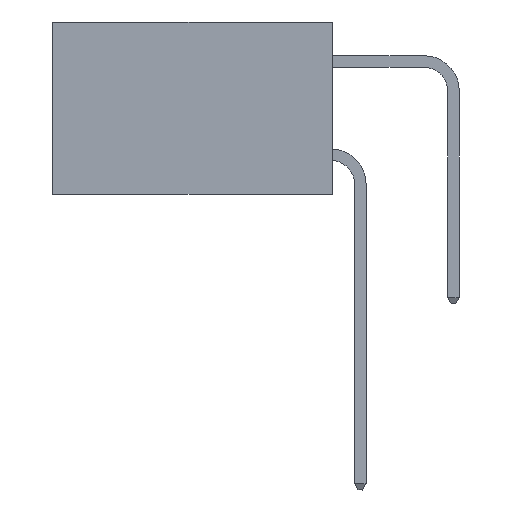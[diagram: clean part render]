
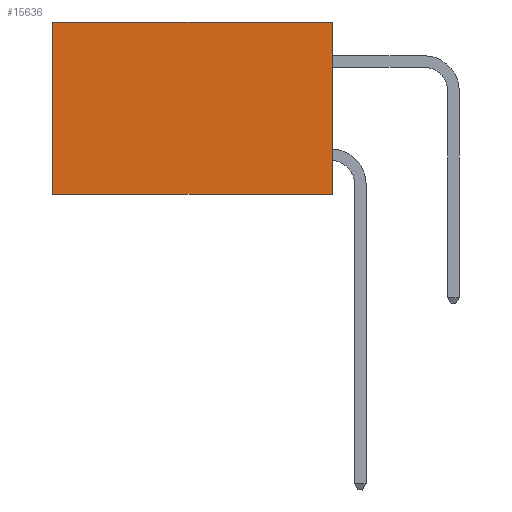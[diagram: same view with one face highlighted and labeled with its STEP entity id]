
A CAD part, left-side view. The second image highlights one B-rep face of the part: STEP entity #15636.
In plain terms, the highlighted planar face has unit normal (-1, 0, 0).
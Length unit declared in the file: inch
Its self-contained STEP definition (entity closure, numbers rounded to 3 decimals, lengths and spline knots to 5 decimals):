
#9 = EDGE_CURVE ( 'NONE', #1922, #20642, #760, .T. ) ;
#76 = EDGE_CURVE ( 'NONE', #8891, #3394, #9156, .T. ) ;
#191 = ORIENTED_EDGE ( 'NONE', *, *, #9, .T. ) ;
#517 = VECTOR ( 'NONE', #4259, 39.37008 ) ;
#760 = LINE ( 'NONE', #12465, #19221 ) ;
#1002 = VECTOR ( 'NONE', #17454, 39.37008 ) ;
#1922 = VERTEX_POINT ( 'NONE', #20510 ) ;
#2182 = AXIS2_PLACEMENT_3D ( 'NONE', #7951, #20433, #9734 ) ;
#2235 = FACE_OUTER_BOUND ( 'NONE', #16258, .T. ) ;
#2481 = CARTESIAN_POINT ( 'NONE',  ( 0.298, 0., 0. ) ) ;
#2521 = PLANE ( 'NONE',  #2182 ) ;
#3394 = VERTEX_POINT ( 'NONE', #10232 ) ;
#4259 = DIRECTION ( 'NONE',  ( 0., 0., -1. ) ) ;
#5754 = CARTESIAN_POINT ( 'NONE',  ( 0.298, 0.6, 0. ) ) ;
#7742 = ORIENTED_EDGE ( 'NONE', *, *, #9142, .T. ) ;
#7951 = CARTESIAN_POINT ( 'NONE',  ( 0.298, 0., 0. ) ) ;
#8891 = VERTEX_POINT ( 'NONE', #18006 ) ;
#9142 = EDGE_CURVE ( 'NONE', #20642, #3394, #10536, .T. ) ;
#9156 = LINE ( 'NONE', #20813, #13301 ) ;
#9257 = DIRECTION ( 'NONE',  ( 0., 1., 0. ) ) ;
#9509 = LINE ( 'NONE', #2481, #517 ) ;
#9734 = DIRECTION ( 'NONE',  ( 0., 0., -1. ) ) ;
#10232 = CARTESIAN_POINT ( 'NONE',  ( 0.298, 0.6, -0.37 ) ) ;
#10536 = LINE ( 'NONE', #5754, #1002 ) ;
#12465 = CARTESIAN_POINT ( 'NONE',  ( 0.298, 0., 0. ) ) ;
#12873 = ORIENTED_EDGE ( 'NONE', *, *, #76, .F. ) ;
#13301 = VECTOR ( 'NONE', #9257, 39.37008 ) ;
#13550 = EDGE_CURVE ( 'NONE', #1922, #8891, #9509, .T. ) ;
#14445 = ORIENTED_EDGE ( 'NONE', *, *, #13550, .F. ) ;
#15636 = ADVANCED_FACE ( 'NONE', ( #2235 ), #2521, .F. ) ;
#15942 = CARTESIAN_POINT ( 'NONE',  ( 0.298, 0.6, 0. ) ) ;
#16258 = EDGE_LOOP ( 'NONE', ( #7742, #12873, #14445, #191 ) ) ;
#17454 = DIRECTION ( 'NONE',  ( 0., 0., -1. ) ) ;
#18006 = CARTESIAN_POINT ( 'NONE',  ( 0.298, 0., -0.37 ) ) ;
#19221 = VECTOR ( 'NONE', #20162, 39.37008 ) ;
#20162 = DIRECTION ( 'NONE',  ( 0., 1., 0. ) ) ;
#20433 = DIRECTION ( 'NONE',  ( 1., 0., 0. ) ) ;
#20510 = CARTESIAN_POINT ( 'NONE',  ( 0.298, 0., 0. ) ) ;
#20642 = VERTEX_POINT ( 'NONE', #15942 ) ;
#20813 = CARTESIAN_POINT ( 'NONE',  ( 0.298, 0., -0.37 ) ) ;
